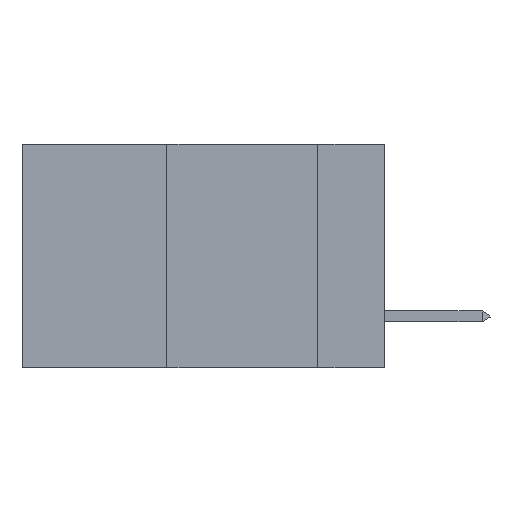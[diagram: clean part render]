
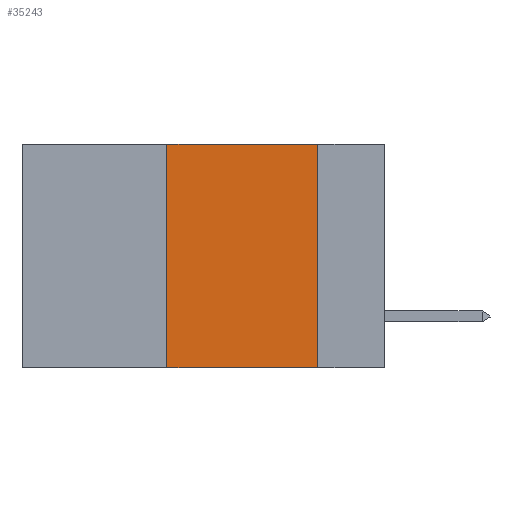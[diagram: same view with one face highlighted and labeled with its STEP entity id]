
A CAD part, left-side view. The second image highlights one B-rep face of the part: STEP entity #35243.
In plain terms, the highlighted planar face has unit normal (-1, 0, 0).
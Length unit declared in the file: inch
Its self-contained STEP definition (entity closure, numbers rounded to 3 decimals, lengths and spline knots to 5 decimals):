
#438 = EDGE_CURVE ( 'NONE', #26963, #21278, #3025, .T. ) ;
#1406 = VECTOR ( 'NONE', #15655, 39.37008 ) ;
#1860 = ORIENTED_EDGE ( 'NONE', *, *, #28858, .F. ) ;
#3025 = LINE ( 'NONE', #28450, #16907 ) ;
#4946 = DIRECTION ( 'NONE',  ( 1., 0., 0. ) ) ;
#7687 = DIRECTION ( 'NONE',  ( 0., 0., -1. ) ) ;
#9783 = EDGE_CURVE ( 'NONE', #26963, #22242, #25011, .T. ) ;
#10388 = CARTESIAN_POINT ( 'NONE',  ( 0., 0.11, -0.37 ) ) ;
#11713 = DIRECTION ( 'NONE',  ( 0., -1., 0. ) ) ;
#11819 = VERTEX_POINT ( 'NONE', #27026 ) ;
#13769 = PLANE ( 'NONE',  #15393 ) ;
#15393 = AXIS2_PLACEMENT_3D ( 'NONE', #16670, #4946, #7687 ) ;
#15655 = DIRECTION ( 'NONE',  ( 0., 0., 1. ) ) ;
#16670 = CARTESIAN_POINT ( 'NONE',  ( 0., 0.6, 0. ) ) ;
#16907 = VECTOR ( 'NONE', #25744, 39.37008 ) ;
#17196 = VECTOR ( 'NONE', #11713, 39.37008 ) ;
#17869 = LINE ( 'NONE', #23748, #34676 ) ;
#20266 = CARTESIAN_POINT ( 'NONE',  ( 0., 0.6, 0. ) ) ;
#21143 = CARTESIAN_POINT ( 'NONE',  ( 0., 0.36, 0. ) ) ;
#21278 = VERTEX_POINT ( 'NONE', #10388 ) ;
#22242 = VERTEX_POINT ( 'NONE', #36734 ) ;
#22320 = ORIENTED_EDGE ( 'NONE', *, *, #9783, .F. ) ;
#23748 = CARTESIAN_POINT ( 'NONE',  ( 0., 0.11, 0. ) ) ;
#23878 = DIRECTION ( 'NONE',  ( 0., 0., -1. ) ) ;
#24066 = FACE_OUTER_BOUND ( 'NONE', #29012, .T. ) ;
#25011 = LINE ( 'NONE', #21143, #1406 ) ;
#25744 = DIRECTION ( 'NONE',  ( 0., -1., 0. ) ) ;
#26963 = VERTEX_POINT ( 'NONE', #29089 ) ;
#27026 = CARTESIAN_POINT ( 'NONE',  ( 0., 0.11, 0. ) ) ;
#27618 = ORIENTED_EDGE ( 'NONE', *, *, #32752, .F. ) ;
#28450 = CARTESIAN_POINT ( 'NONE',  ( 0., 0.6, -0.37 ) ) ;
#28858 = EDGE_CURVE ( 'NONE', #11819, #21278, #17869, .T. ) ;
#29012 = EDGE_LOOP ( 'NONE', ( #1860, #27618, #22320, #29566 ) ) ;
#29089 = CARTESIAN_POINT ( 'NONE',  ( 0., 0.36, -0.37 ) ) ;
#29566 = ORIENTED_EDGE ( 'NONE', *, *, #438, .T. ) ;
#29613 = LINE ( 'NONE', #20266, #17196 ) ;
#32752 = EDGE_CURVE ( 'NONE', #22242, #11819, #29613, .T. ) ;
#34676 = VECTOR ( 'NONE', #23878, 39.37008 ) ;
#35243 = ADVANCED_FACE ( 'NONE', ( #24066 ), #13769, .F. ) ;
#36734 = CARTESIAN_POINT ( 'NONE',  ( 0., 0.36, 0. ) ) ;
